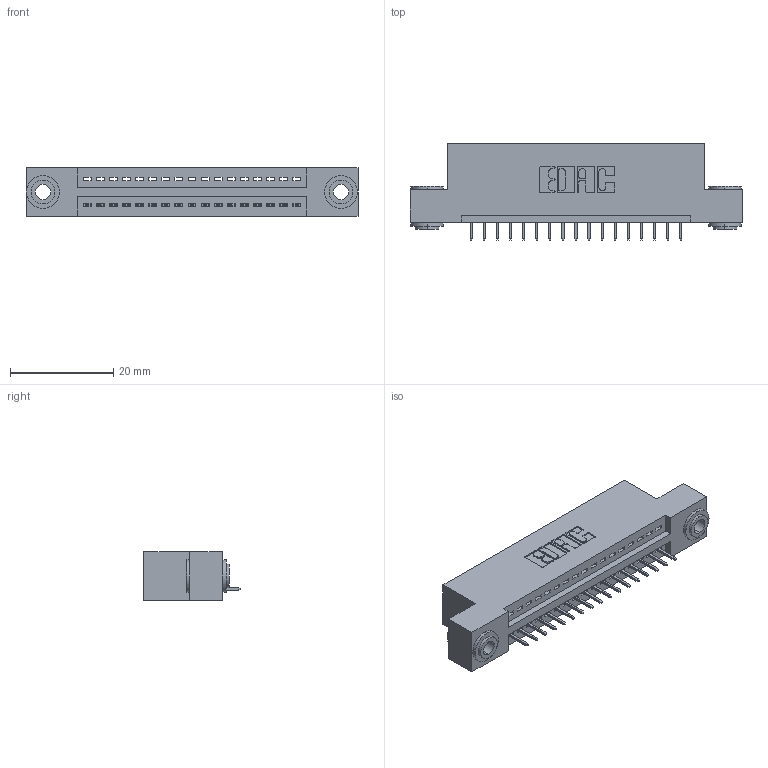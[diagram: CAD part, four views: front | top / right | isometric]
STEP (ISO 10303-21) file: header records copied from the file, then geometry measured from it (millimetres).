
FILE_DESCRIPTION (( 'STEP AP203' ), '1' );
FILE_NAME ('895-017-525-103.STEP', '2020-09-25T05:36:28', ( '' ), ( '' ), 'SwSTEP 2.0', 'SolidWorks 2020', '' );
FILE_SCHEMA (( 'CONFIG_CONTROL_DESIGN' ));
Length unit declared in the file: inch
Products named in the file (4): 845 Part_Flush Mounting Lugs - 0.156 Dia-TH; 895-017-525-103; 345-292-001_345-293-125; 345-250-002_345-250-002-102
Assembly tree (20 placements, depth 2):
  895-017-525-103
    845 Part_Flush Mounting Lugs - 0.156 Dia-TH
    345-292-001_345-293-125  x17
    345-250-002_345-250-002-102  x2
Bounding box: 64.39 x 18.72 x 9.4 mm (x, y, z)
Volume: 5860.9 mm3; surface area: 7431.9 mm2
Topology: 20 solids, 20 shells, 1218 faces, 3477 edges, 2246 vertices
Faces by surface type: plane 872, cylinder 338, cone 8
Entity records: 16884 total; most frequent: CARTESIAN_POINT 2902, ORIENTED_EDGE 2846, DIRECTION 2603, EDGE_CURVE 1423, VECTOR 1203, LINE 1203, VERTEX_POINT 942, AXIS2_PLACEMENT_3D 700
